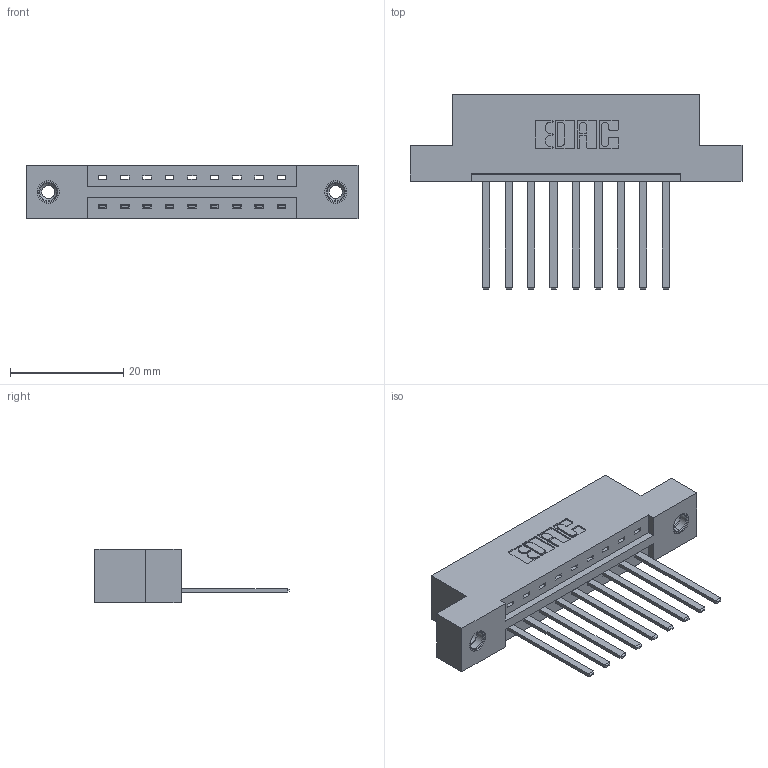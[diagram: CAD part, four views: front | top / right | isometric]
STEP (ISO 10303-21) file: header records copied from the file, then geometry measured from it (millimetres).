
FILE_DESCRIPTION (( 'STEP AP203' ), '1' );
FILE_NAME ('387-009-544-108.STEP', '2019-10-02T10:48:56', ( '' ), ( '' ), 'SwSTEP 2.0', 'SolidWorks 2016', '' );
FILE_SCHEMA (( 'CONFIG_CONTROL_DESIGN' ));
Length unit declared in the file: inch
Products named in the file (4): 345-292-001_345-293-144; 387-009-544-108; 337 Part_Flush Mounting Lugs - 0.156 Dia-TI; 345-250-001_345-250-003-102
Assembly tree (12 placements, depth 2):
  387-009-544-108
    337 Part_Flush Mounting Lugs - 0.156 Dia-TI
    345-292-001_345-293-144  x9
    345-250-001_345-250-003-102  x2
Bounding box: 58.67 x 34.3 x 9.4 mm (x, y, z)
Volume: 5782.9 mm3; surface area: 6165.2 mm2
Topology: 12 solids, 12 shells, 678 faces, 1977 edges, 1298 vertices
Faces by surface type: plane 480, cylinder 182, cone 12, torus 4
Entity records: 11960 total; most frequent: CARTESIAN_POINT 2060, ORIENTED_EDGE 1998, DIRECTION 1831, EDGE_CURVE 999, VECTOR 855, LINE 855, VERTEX_POINT 660, AXIS2_PLACEMENT_3D 488
